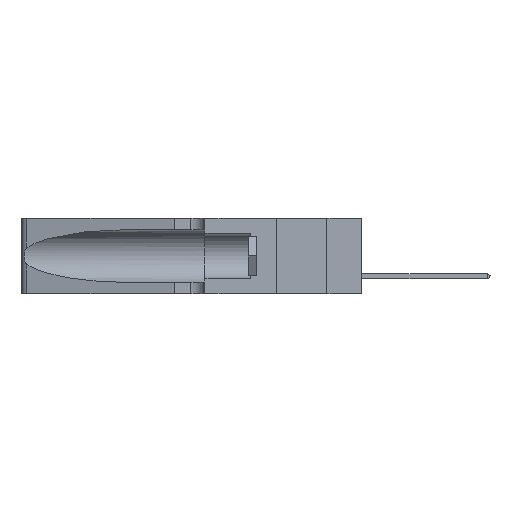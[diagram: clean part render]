
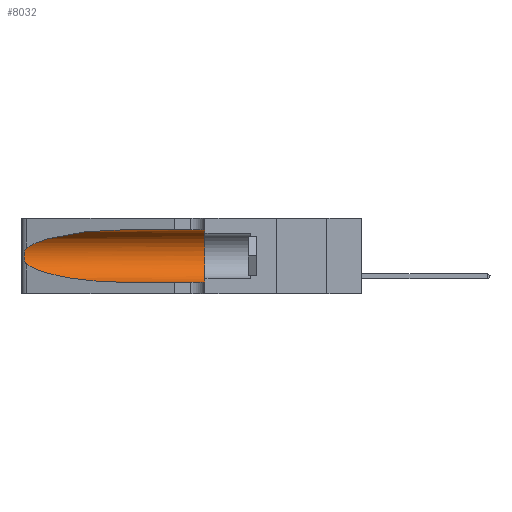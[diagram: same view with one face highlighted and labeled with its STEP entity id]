
A CAD part, left-side view. The second image highlights one B-rep face of the part: STEP entity #8032.
In plain terms, the highlighted cylindrical face has radius 3.308 mm (diameter 6.617 mm), a partial arc.
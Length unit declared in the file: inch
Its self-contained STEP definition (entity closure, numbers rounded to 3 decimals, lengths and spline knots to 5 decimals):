
#638 = CARTESIAN_POINT ( 'NONE',  ( 0.25854, 1.2359, 0.20912 ) ) ;
#2224 =( BOUNDED_CURVE ( )  B_SPLINE_CURVE ( 3, ( #18484, #15246, #23821, #26788 ),
 .UNSPECIFIED., .F., .F. ) 
 B_SPLINE_CURVE_WITH_KNOTS ( ( 4, 4 ),
 ( 3.44316, 4.71239 ),
 .UNSPECIFIED. ) 
 CURVE ( )  GEOMETRIC_REPRESENTATION_ITEM ( )  RATIONAL_B_SPLINE_CURVE ( ( 1., 0.87, 0.87, 1. ) ) 
 REPRESENTATION_ITEM ( '' )  );
#6143 = EDGE_CURVE ( 'NONE', #28913, #14863, #22029, .T. ) ;
#6626 = CARTESIAN_POINT ( 'NONE',  ( 0.26017, 1.23833, 0.17102 ) ) ;
#6746 = CARTESIAN_POINT ( 'NONE',  ( 0.25555, 1.22994, 0.2215 ) ) ;
#7368 = CARTESIAN_POINT ( 'NONE',  ( 0.18966, 0.96281, 0.31525 ) ) ;
#7904 = EDGE_CURVE ( 'NONE', #28913, #14325, #28991, .T. ) ;
#8032 = ADVANCED_FACE ( 'NONE', ( #30730 ), #21514, .F. ) ;
#8749 = VECTOR ( 'NONE', #13484, 39.37008 ) ;
#9453 = VERTEX_POINT ( 'NONE', #20593 ) ;
#11574 = VERTEX_POINT ( 'NONE', #23476 ) ;
#12537 = CARTESIAN_POINT ( 'NONE',  ( 0.26018, 1.23835, 0.19895 ) ) ;
#12679 = CARTESIAN_POINT ( 'NONE',  ( 0.25639, 1.23184, 0.21858 ) ) ;
#12947 = CARTESIAN_POINT ( 'NONE',  ( 0.25856, 1.23593, 0.16098 ) ) ;
#13484 = DIRECTION ( 'NONE',  ( 0., -1., 0. ) ) ;
#14325 = VERTEX_POINT ( 'NONE', #31631 ) ;
#14486 = ORIENTED_EDGE ( 'NONE', *, *, #32698, .T. ) ;
#14863 = VERTEX_POINT ( 'NONE', #20751 ) ;
#15232 = CIRCLE ( 'NONE', #20752, 0.13025 ) ;
#15246 = CARTESIAN_POINT ( 'NONE',  ( 0.2373, 1.15595, 0.08982 ) ) ;
#16769 = EDGE_LOOP ( 'NONE', ( #24106, #19066, #16832, #14486, #20333, #34155 ) ) ;
#16832 = ORIENTED_EDGE ( 'NONE', *, *, #34480, .T. ) ;
#16874 = EDGE_CURVE ( 'NONE', #14863, #9453, #17125, .T. ) ;
#17125 = B_SPLINE_CURVE_WITH_KNOTS ( 'NONE', 3,
 ( #18353, #6746, #12679, #21397, #638, #12537, #21534, #24193, #6626, #12947, #36551, #33006, #33552, #27611 ),
 .UNSPECIFIED., .F., .F.,
 ( 4, 2, 2, 2, 2, 2, 4 ),
 ( 0., 0.00027, 0.00053, 0.00107, 0.0016, 0.00187, 0.00214 ),
 .UNSPECIFIED. ) ;
#18353 = CARTESIAN_POINT ( 'NONE',  ( 0.25487, 1.22718, 0.22369 ) ) ;
#18484 = CARTESIAN_POINT ( 'NONE',  ( 0.25487, 1.22718, 0.14631 ) ) ;
#19008 = CARTESIAN_POINT ( 'NONE',  ( 0.1305, 1.61858, 0.05475 ) ) ;
#19066 = ORIENTED_EDGE ( 'NONE', *, *, #16874, .T. ) ;
#19365 = CARTESIAN_POINT ( 'NONE',  ( 0.2373, 1.15595, 0.28018 ) ) ;
#19495 = CARTESIAN_POINT ( 'NONE',  ( 0.25487, 1.22718, 0.22369 ) ) ;
#20223 = LINE ( 'NONE', #19008, #8749 ) ;
#20333 = ORIENTED_EDGE ( 'NONE', *, *, #27248, .F. ) ;
#20593 = CARTESIAN_POINT ( 'NONE',  ( 0.25487, 1.22718, 0.14631 ) ) ;
#20751 = CARTESIAN_POINT ( 'NONE',  ( 0.25487, 1.22718, 0.22369 ) ) ;
#20752 = AXIS2_PLACEMENT_3D ( 'NONE', #32847, #26908, #20991 ) ;
#20991 = DIRECTION ( 'NONE',  ( 0., 0., 1. ) ) ;
#21397 = CARTESIAN_POINT ( 'NONE',  ( 0.25787, 1.23484, 0.2124 ) ) ;
#21514 = CYLINDRICAL_SURFACE ( 'NONE', #33067, 0.13025 ) ;
#21534 = CARTESIAN_POINT ( 'NONE',  ( 0.26075, 1.23896, 0.19203 ) ) ;
#22029 =( BOUNDED_CURVE ( )  B_SPLINE_CURVE ( 3, ( #33621, #7368, #19365, #19495 ),
 .UNSPECIFIED., .F., .F. ) 
 B_SPLINE_CURVE_WITH_KNOTS ( ( 4, 4 ),
 ( 1.5708, 2.84003 ),
 .UNSPECIFIED. ) 
 CURVE ( )  GEOMETRIC_REPRESENTATION_ITEM ( )  RATIONAL_B_SPLINE_CURVE ( ( 1., 0.87, 0.87, 1. ) ) 
 REPRESENTATION_ITEM ( '' )  );
#23159 = CARTESIAN_POINT ( 'NONE',  ( 0.1305, 1.61858, 0.185 ) ) ;
#23476 = CARTESIAN_POINT ( 'NONE',  ( 0.1305, 0.35, 0.05475 ) ) ;
#23821 = CARTESIAN_POINT ( 'NONE',  ( 0.18966, 0.96281, 0.05475 ) ) ;
#24106 = ORIENTED_EDGE ( 'NONE', *, *, #6143, .T. ) ;
#24193 = CARTESIAN_POINT ( 'NONE',  ( 0.26075, 1.23896, 0.178 ) ) ;
#26788 = CARTESIAN_POINT ( 'NONE',  ( 0.1305, 0.72297, 0.05475 ) ) ;
#26908 = DIRECTION ( 'NONE',  ( 0., 1., 0. ) ) ;
#27248 = EDGE_CURVE ( 'NONE', #14325, #11574, #15232, .T. ) ;
#27611 = CARTESIAN_POINT ( 'NONE',  ( 0.25487, 1.22718, 0.14631 ) ) ;
#27703 = CARTESIAN_POINT ( 'NONE',  ( 0.1305, 0.72297, 0.31525 ) ) ;
#28449 = CARTESIAN_POINT ( 'NONE',  ( 0.1305, 0.72297, 0.05475 ) ) ;
#28913 = VERTEX_POINT ( 'NONE', #27703 ) ;
#28991 = LINE ( 'NONE', #33337, #32598 ) ;
#28994 = DIRECTION ( 'NONE',  ( 0., -1., 0. ) ) ;
#30730 = FACE_OUTER_BOUND ( 'NONE', #16769, .T. ) ;
#31631 = CARTESIAN_POINT ( 'NONE',  ( 0.1305, 0.35, 0.31525 ) ) ;
#32598 = VECTOR ( 'NONE', #36745, 39.37008 ) ;
#32698 = EDGE_CURVE ( 'NONE', #37938, #11574, #20223, .T. ) ;
#32847 = CARTESIAN_POINT ( 'NONE',  ( 0.1305, 0.35, 0.185 ) ) ;
#33006 = CARTESIAN_POINT ( 'NONE',  ( 0.25639, 1.23186, 0.15144 ) ) ;
#33067 = AXIS2_PLACEMENT_3D ( 'NONE', #23159, #28994, #38057 ) ;
#33337 = CARTESIAN_POINT ( 'NONE',  ( 0.1305, 1.61858, 0.31525 ) ) ;
#33552 = CARTESIAN_POINT ( 'NONE',  ( 0.25555, 1.22993, 0.14849 ) ) ;
#33621 = CARTESIAN_POINT ( 'NONE',  ( 0.1305, 0.72297, 0.31525 ) ) ;
#34155 = ORIENTED_EDGE ( 'NONE', *, *, #7904, .F. ) ;
#34480 = EDGE_CURVE ( 'NONE', #9453, #37938, #2224, .T. ) ;
#36551 = CARTESIAN_POINT ( 'NONE',  ( 0.25789, 1.23486, 0.15765 ) ) ;
#36745 = DIRECTION ( 'NONE',  ( 0., -1., 0. ) ) ;
#37938 = VERTEX_POINT ( 'NONE', #28449 ) ;
#38057 = DIRECTION ( 'NONE',  ( 0., 0., -1. ) ) ;
